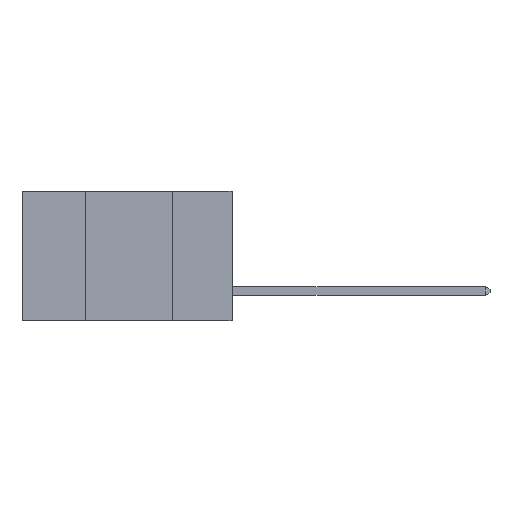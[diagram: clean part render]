
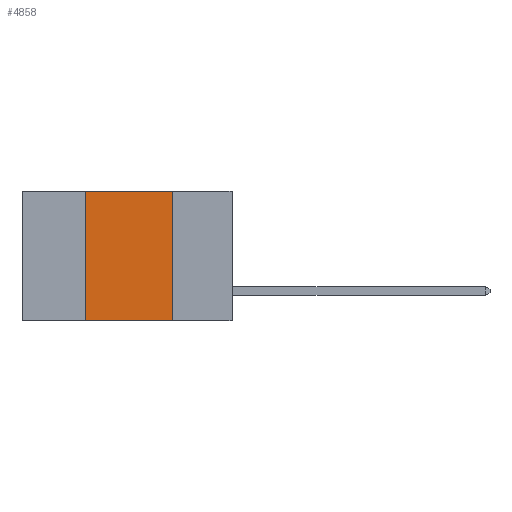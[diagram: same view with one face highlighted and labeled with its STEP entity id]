
A CAD part, left-side view. The second image highlights one B-rep face of the part: STEP entity #4858.
In plain terms, the highlighted planar face has unit normal (-1, 0, 0).
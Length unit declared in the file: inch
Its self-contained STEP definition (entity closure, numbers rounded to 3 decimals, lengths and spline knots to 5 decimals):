
#172 = PLANE ( 'NONE',  #6205 ) ;
#247 = CARTESIAN_POINT ( 'NONE',  ( 0., 0.17, -0.37 ) ) ;
#280 = CARTESIAN_POINT ( 'NONE',  ( 0., 0.17, 0. ) ) ;
#1124 = LINE ( 'NONE', #280, #7540 ) ;
#1333 = CARTESIAN_POINT ( 'NONE',  ( 0., 0.42, -0.37 ) ) ;
#2364 = VERTEX_POINT ( 'NONE', #247 ) ;
#2831 = DIRECTION ( 'NONE',  ( 0., -1., 0. ) ) ;
#3260 = VERTEX_POINT ( 'NONE', #8594 ) ;
#3428 = EDGE_LOOP ( 'NONE', ( #6196, #7590, #15367, #7203 ) ) ;
#3958 = DIRECTION ( 'NONE',  ( 1., 0., 0. ) ) ;
#4042 = VECTOR ( 'NONE', #10941, 39.37008 ) ;
#4608 = CARTESIAN_POINT ( 'NONE',  ( 0., 0.6, 0. ) ) ;
#4858 = ADVANCED_FACE ( 'NONE', ( #5972 ), #172, .F. ) ;
#5277 = VECTOR ( 'NONE', #6005, 39.37008 ) ;
#5796 = VERTEX_POINT ( 'NONE', #1333 ) ;
#5972 = FACE_OUTER_BOUND ( 'NONE', #3428, .T. ) ;
#6005 = DIRECTION ( 'NONE',  ( 0., 0., 1. ) ) ;
#6196 = ORIENTED_EDGE ( 'NONE', *, *, #16238, .F. ) ;
#6205 = AXIS2_PLACEMENT_3D ( 'NONE', #15278, #3958, #9082 ) ;
#7077 = LINE ( 'NONE', #4608, #4042 ) ;
#7203 = ORIENTED_EDGE ( 'NONE', *, *, #7761, .T. ) ;
#7540 = VECTOR ( 'NONE', #10466, 39.37008 ) ;
#7590 = ORIENTED_EDGE ( 'NONE', *, *, #8483, .F. ) ;
#7761 = EDGE_CURVE ( 'NONE', #5796, #2364, #14861, .T. ) ;
#7944 = CARTESIAN_POINT ( 'NONE',  ( 0., 0.6, -0.37 ) ) ;
#8483 = EDGE_CURVE ( 'NONE', #9353, #3260, #7077, .T. ) ;
#8594 = CARTESIAN_POINT ( 'NONE',  ( 0., 0.17, 0. ) ) ;
#9082 = DIRECTION ( 'NONE',  ( 0., 0., -1. ) ) ;
#9353 = VERTEX_POINT ( 'NONE', #11461 ) ;
#10466 = DIRECTION ( 'NONE',  ( 0., 0., -1. ) ) ;
#10941 = DIRECTION ( 'NONE',  ( 0., -1., 0. ) ) ;
#11461 = CARTESIAN_POINT ( 'NONE',  ( 0., 0.42, 0. ) ) ;
#11593 = VECTOR ( 'NONE', #2831, 39.37008 ) ;
#11946 = EDGE_CURVE ( 'NONE', #5796, #9353, #15636, .T. ) ;
#13532 = CARTESIAN_POINT ( 'NONE',  ( 0., 0.42, 0. ) ) ;
#14861 = LINE ( 'NONE', #7944, #11593 ) ;
#15278 = CARTESIAN_POINT ( 'NONE',  ( 0., 0.6, 0. ) ) ;
#15367 = ORIENTED_EDGE ( 'NONE', *, *, #11946, .F. ) ;
#15636 = LINE ( 'NONE', #13532, #5277 ) ;
#16238 = EDGE_CURVE ( 'NONE', #3260, #2364, #1124, .T. ) ;
